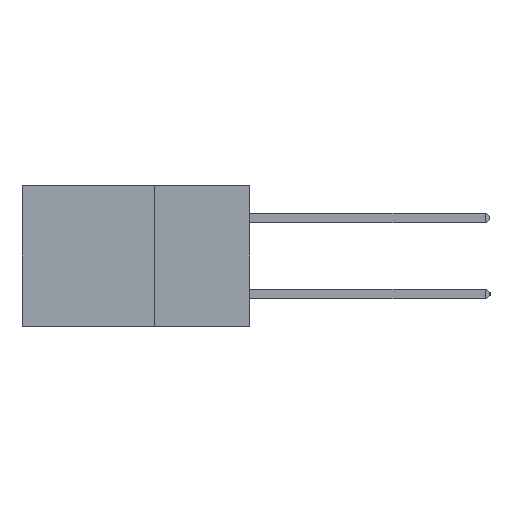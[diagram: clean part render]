
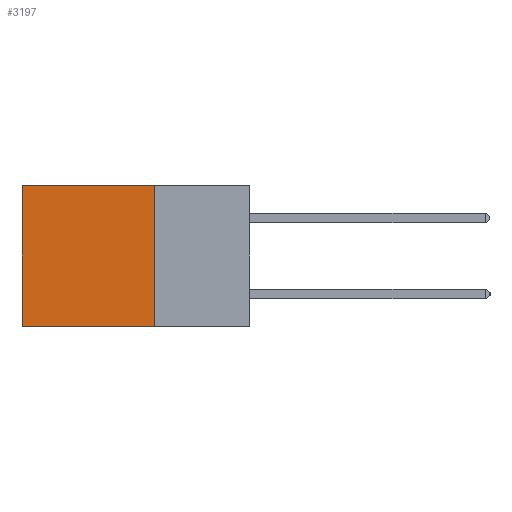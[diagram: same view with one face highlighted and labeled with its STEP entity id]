
A CAD part, left-side view. The second image highlights one B-rep face of the part: STEP entity #3197.
In plain terms, the highlighted planar face has unit normal (-1, 0, 0).
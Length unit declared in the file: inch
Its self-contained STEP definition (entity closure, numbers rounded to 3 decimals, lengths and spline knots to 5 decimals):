
#82 = EDGE_CURVE ( 'NONE', #10192, #6173, #13238, .T. ) ;
#294 = LINE ( 'NONE', #4037, #11217 ) ;
#614 = CARTESIAN_POINT ( 'NONE',  ( 0.2875, 0.25, -0.37 ) ) ;
#1734 = DIRECTION ( 'NONE',  ( 0., 0., -1. ) ) ;
#1887 = EDGE_CURVE ( 'NONE', #6173, #1947, #5558, .T. ) ;
#1923 = ORIENTED_EDGE ( 'NONE', *, *, #3398, .T. ) ;
#1947 = VERTEX_POINT ( 'NONE', #2011 ) ;
#1979 = VECTOR ( 'NONE', #5394, 39.37008 ) ;
#2011 = CARTESIAN_POINT ( 'NONE',  ( 0.2875, 0.6, -0.37 ) ) ;
#2156 = PLANE ( 'NONE',  #3025 ) ;
#2344 = VECTOR ( 'NONE', #5512, 39.37008 ) ;
#2783 = VERTEX_POINT ( 'NONE', #4127 ) ;
#2996 = EDGE_LOOP ( 'NONE', ( #1923, #5086, #7729, #10212 ) ) ;
#3025 = AXIS2_PLACEMENT_3D ( 'NONE', #12374, #3374, #10463 ) ;
#3197 = ADVANCED_FACE ( 'NONE', ( #12253 ), #2156, .F. ) ;
#3374 = DIRECTION ( 'NONE',  ( 1., 0., 0. ) ) ;
#3398 = EDGE_CURVE ( 'NONE', #2783, #1947, #5506, .T. ) ;
#4037 = CARTESIAN_POINT ( 'NONE',  ( 0.2875, 0.25, 0. ) ) ;
#4127 = CARTESIAN_POINT ( 'NONE',  ( 0.2875, 0.6, 0. ) ) ;
#5086 = ORIENTED_EDGE ( 'NONE', *, *, #1887, .F. ) ;
#5394 = DIRECTION ( 'NONE',  ( 0., 0., -1. ) ) ;
#5506 = LINE ( 'NONE', #10146, #1979 ) ;
#5512 = DIRECTION ( 'NONE',  ( 0., 1., 0. ) ) ;
#5558 = LINE ( 'NONE', #614, #2344 ) ;
#6173 = VERTEX_POINT ( 'NONE', #10746 ) ;
#7565 = CARTESIAN_POINT ( 'NONE',  ( 0.2875, 0.25, 0. ) ) ;
#7729 = ORIENTED_EDGE ( 'NONE', *, *, #82, .F. ) ;
#10146 = CARTESIAN_POINT ( 'NONE',  ( 0.2875, 0.6, 0. ) ) ;
#10192 = VERTEX_POINT ( 'NONE', #7565 ) ;
#10212 = ORIENTED_EDGE ( 'NONE', *, *, #12023, .T. ) ;
#10375 = VECTOR ( 'NONE', #1734, 39.37008 ) ;
#10463 = DIRECTION ( 'NONE',  ( 0., 0., -1. ) ) ;
#10490 = CARTESIAN_POINT ( 'NONE',  ( 0.2875, 0.25, 0. ) ) ;
#10746 = CARTESIAN_POINT ( 'NONE',  ( 0.2875, 0.25, -0.37 ) ) ;
#11217 = VECTOR ( 'NONE', #11967, 39.37008 ) ;
#11967 = DIRECTION ( 'NONE',  ( 0., 1., 0. ) ) ;
#12023 = EDGE_CURVE ( 'NONE', #10192, #2783, #294, .T. ) ;
#12253 = FACE_OUTER_BOUND ( 'NONE', #2996, .T. ) ;
#12374 = CARTESIAN_POINT ( 'NONE',  ( 0.2875, 0.25, 0. ) ) ;
#13238 = LINE ( 'NONE', #10490, #10375 ) ;
